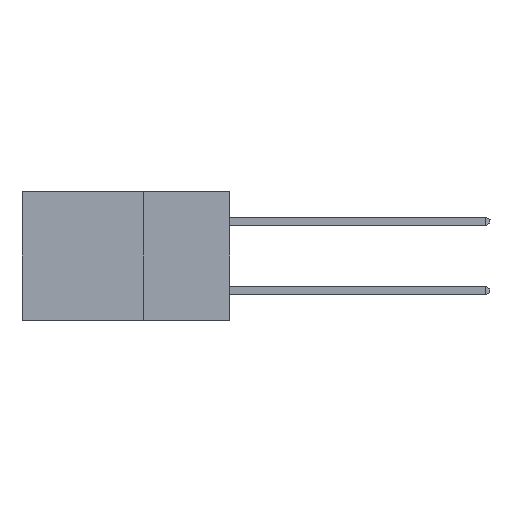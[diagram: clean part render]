
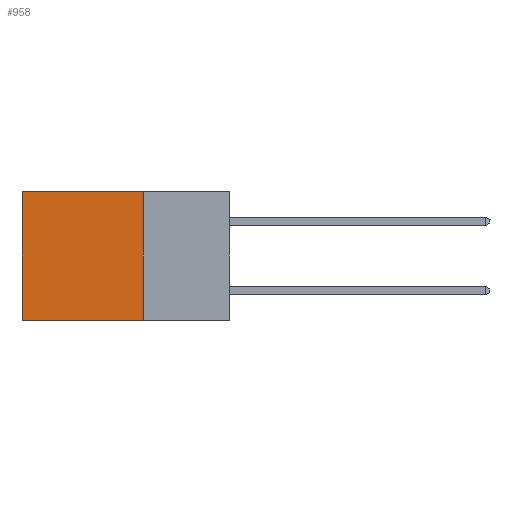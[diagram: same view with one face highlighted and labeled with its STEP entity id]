
A CAD part, left-side view. The second image highlights one B-rep face of the part: STEP entity #958.
In plain terms, the highlighted planar face has unit normal (-1, 0, 0).
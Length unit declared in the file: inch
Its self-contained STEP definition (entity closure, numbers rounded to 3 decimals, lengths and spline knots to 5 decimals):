
#332 = EDGE_CURVE ( 'NONE', #16727, #7723, #16576, .T. ) ;
#400 = LINE ( 'NONE', #7426, #22296 ) ;
#958 = ADVANCED_FACE ( 'NONE', ( #9249 ), #16770, .F. ) ;
#1142 = VECTOR ( 'NONE', #3036, 39.37008 ) ;
#2254 = CARTESIAN_POINT ( 'NONE',  ( 0.298, 0.25, -0.37 ) ) ;
#3036 = DIRECTION ( 'NONE',  ( 0., 0., -1. ) ) ;
#3439 = EDGE_LOOP ( 'NONE', ( #24911, #4123, #15022, #15555 ) ) ;
#4123 = ORIENTED_EDGE ( 'NONE', *, *, #332, .F. ) ;
#4467 = VERTEX_POINT ( 'NONE', #20706 ) ;
#6128 = CARTESIAN_POINT ( 'NONE',  ( 0.298, 0.25, -0.37 ) ) ;
#6170 = EDGE_CURVE ( 'NONE', #7692, #7723, #24499, .T. ) ;
#7426 = CARTESIAN_POINT ( 'NONE',  ( 0.298, 0.25, 0. ) ) ;
#7692 = VERTEX_POINT ( 'NONE', #15917 ) ;
#7723 = VERTEX_POINT ( 'NONE', #20258 ) ;
#8738 = EDGE_CURVE ( 'NONE', #4467, #7692, #400, .T. ) ;
#9092 = DIRECTION ( 'NONE',  ( 1., 0., 0. ) ) ;
#9249 = FACE_OUTER_BOUND ( 'NONE', #3439, .T. ) ;
#9550 = DIRECTION ( 'NONE',  ( 0., 1., 0. ) ) ;
#11025 = AXIS2_PLACEMENT_3D ( 'NONE', #21570, #9092, #23968 ) ;
#12282 = VECTOR ( 'NONE', #19264, 39.37008 ) ;
#13780 = CARTESIAN_POINT ( 'NONE',  ( 0.298, 0.25, 0. ) ) ;
#15022 = ORIENTED_EDGE ( 'NONE', *, *, #22011, .F. ) ;
#15555 = ORIENTED_EDGE ( 'NONE', *, *, #8738, .T. ) ;
#15850 = VECTOR ( 'NONE', #16536, 39.37008 ) ;
#15917 = CARTESIAN_POINT ( 'NONE',  ( 0.298, 0.6, 0. ) ) ;
#16536 = DIRECTION ( 'NONE',  ( 0., 0., -1. ) ) ;
#16576 = LINE ( 'NONE', #2254, #12282 ) ;
#16727 = VERTEX_POINT ( 'NONE', #6128 ) ;
#16770 = PLANE ( 'NONE',  #11025 ) ;
#19157 = CARTESIAN_POINT ( 'NONE',  ( 0.298, 0.6, 0. ) ) ;
#19264 = DIRECTION ( 'NONE',  ( 0., 1., 0. ) ) ;
#20258 = CARTESIAN_POINT ( 'NONE',  ( 0.298, 0.6, -0.37 ) ) ;
#20706 = CARTESIAN_POINT ( 'NONE',  ( 0.298, 0.25, 0. ) ) ;
#21570 = CARTESIAN_POINT ( 'NONE',  ( 0.298, 0.25, 0. ) ) ;
#22011 = EDGE_CURVE ( 'NONE', #4467, #16727, #27278, .T. ) ;
#22296 = VECTOR ( 'NONE', #9550, 39.37008 ) ;
#23968 = DIRECTION ( 'NONE',  ( 0., 0., -1. ) ) ;
#24499 = LINE ( 'NONE', #19157, #15850 ) ;
#24911 = ORIENTED_EDGE ( 'NONE', *, *, #6170, .T. ) ;
#27278 = LINE ( 'NONE', #13780, #1142 ) ;
